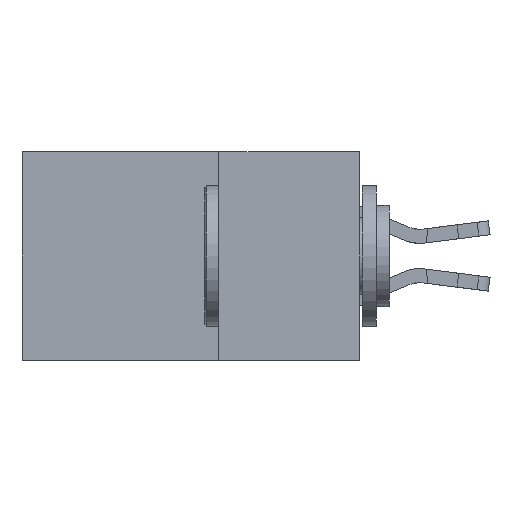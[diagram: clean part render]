
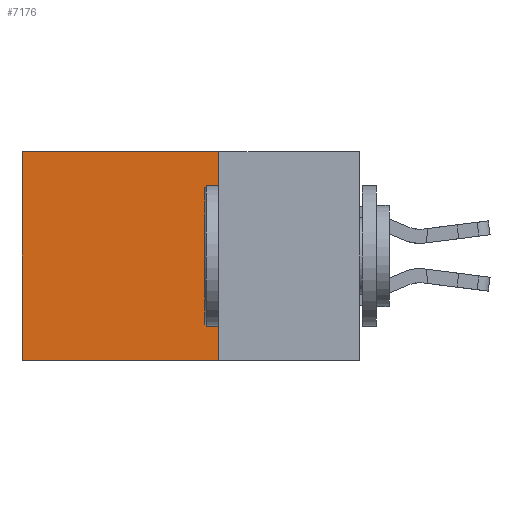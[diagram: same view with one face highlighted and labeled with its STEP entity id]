
A CAD part, left-side view. The second image highlights one B-rep face of the part: STEP entity #7176.
In plain terms, the highlighted planar face has unit normal (-1, 0, 0).
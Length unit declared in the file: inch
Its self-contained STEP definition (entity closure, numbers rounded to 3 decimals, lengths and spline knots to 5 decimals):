
#470 = CARTESIAN_POINT ( 'NONE',  ( 0.2875, 0.25, 0. ) ) ;
#1778 = EDGE_CURVE ( 'NONE', #31884, #4284, #5800, .T. ) ;
#4284 = VERTEX_POINT ( 'NONE', #21589 ) ;
#5207 = FACE_OUTER_BOUND ( 'NONE', #35476, .T. ) ;
#5800 = LINE ( 'NONE', #30205, #25721 ) ;
#6449 = DIRECTION ( 'NONE',  ( 0., 0., -1. ) ) ;
#7176 = ADVANCED_FACE ( 'NONE', ( #5207 ), #31249, .F. ) ;
#7460 = CARTESIAN_POINT ( 'NONE',  ( 0.2875, 0.25, 0. ) ) ;
#7518 = LINE ( 'NONE', #10192, #34358 ) ;
#8408 = EDGE_CURVE ( 'NONE', #23010, #31884, #22799, .T. ) ;
#8856 = DIRECTION ( 'NONE',  ( 1., 0., 0. ) ) ;
#10192 = CARTESIAN_POINT ( 'NONE',  ( 0.2875, 0.25, 0. ) ) ;
#12004 = ORIENTED_EDGE ( 'NONE', *, *, #14175, .F. ) ;
#14175 = EDGE_CURVE ( 'NONE', #27765, #4284, #14886, .T. ) ;
#14233 = DIRECTION ( 'NONE',  ( 0., 1., 0. ) ) ;
#14886 = LINE ( 'NONE', #23527, #35238 ) ;
#15463 = VECTOR ( 'NONE', #14233, 39.37008 ) ;
#16553 = ORIENTED_EDGE ( 'NONE', *, *, #8408, .T. ) ;
#19099 = AXIS2_PLACEMENT_3D ( 'NONE', #470, #8856, #6449 ) ;
#21089 = ORIENTED_EDGE ( 'NONE', *, *, #31375, .F. ) ;
#21153 = DIRECTION ( 'NONE',  ( 0., 0., -1. ) ) ;
#21589 = CARTESIAN_POINT ( 'NONE',  ( 0.2875, 0.6, -0.37 ) ) ;
#22799 = LINE ( 'NONE', #33471, #15463 ) ;
#23010 = VERTEX_POINT ( 'NONE', #7460 ) ;
#23527 = CARTESIAN_POINT ( 'NONE',  ( 0.2875, 0.25, -0.37 ) ) ;
#23648 = DIRECTION ( 'NONE',  ( 0., 1., 0. ) ) ;
#23715 = CARTESIAN_POINT ( 'NONE',  ( 0.2875, 0.6, 0. ) ) ;
#25721 = VECTOR ( 'NONE', #27281, 39.37008 ) ;
#27281 = DIRECTION ( 'NONE',  ( 0., 0., -1. ) ) ;
#27765 = VERTEX_POINT ( 'NONE', #31781 ) ;
#30205 = CARTESIAN_POINT ( 'NONE',  ( 0.2875, 0.6, 0. ) ) ;
#31249 = PLANE ( 'NONE',  #19099 ) ;
#31375 = EDGE_CURVE ( 'NONE', #23010, #27765, #7518, .T. ) ;
#31781 = CARTESIAN_POINT ( 'NONE',  ( 0.2875, 0.25, -0.37 ) ) ;
#31884 = VERTEX_POINT ( 'NONE', #23715 ) ;
#33471 = CARTESIAN_POINT ( 'NONE',  ( 0.2875, 0.25, 0. ) ) ;
#34358 = VECTOR ( 'NONE', #21153, 39.37008 ) ;
#35238 = VECTOR ( 'NONE', #23648, 39.37008 ) ;
#35476 = EDGE_LOOP ( 'NONE', ( #35594, #12004, #21089, #16553 ) ) ;
#35594 = ORIENTED_EDGE ( 'NONE', *, *, #1778, .T. ) ;
